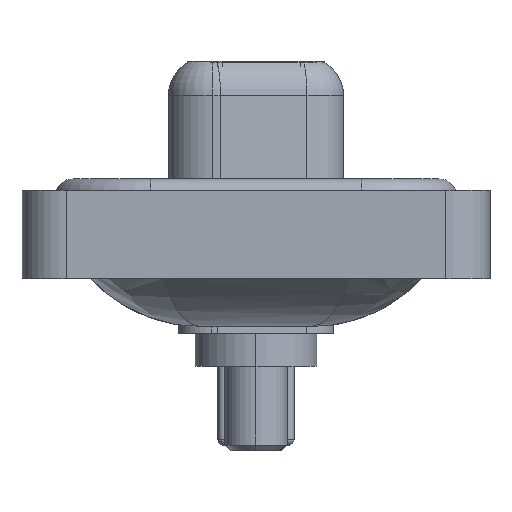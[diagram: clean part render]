
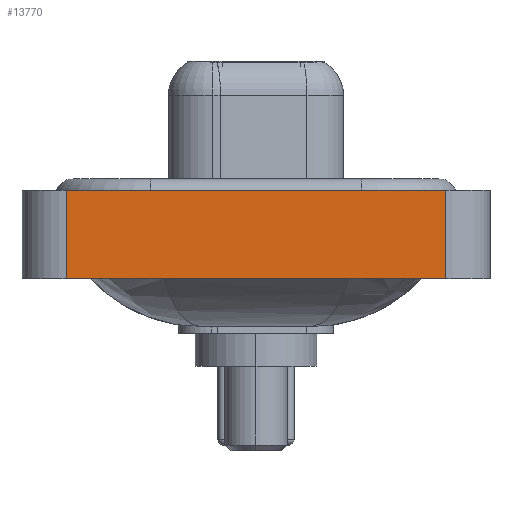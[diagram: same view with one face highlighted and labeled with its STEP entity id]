
A CAD part, left-side view. The second image highlights one B-rep face of the part: STEP entity #13770.
In plain terms, the highlighted planar face has unit normal (-1, 0, 0).
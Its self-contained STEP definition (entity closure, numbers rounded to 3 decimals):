
#622 = EDGE_CURVE ( 'NONE', #10113, #8779, #14927, .T. ) ;
#1394 = DIRECTION ( 'NONE',  ( 0., -1., 0. ) ) ;
#2522 = DIRECTION ( 'NONE',  ( -1., 0., 0. ) ) ;
#2656 = CARTESIAN_POINT ( 'NONE',  ( -7.35, -8.55, -3.6 ) ) ;
#2836 = DIRECTION ( 'NONE',  ( 0., -1., 0. ) ) ;
#3426 = VECTOR ( 'NONE', #14738, 1000. ) ;
#4171 = CARTESIAN_POINT ( 'NONE',  ( -7.35, 8.55, -3.6 ) ) ;
#4518 = ORIENTED_EDGE ( 'NONE', *, *, #9987, .F. ) ;
#4625 = CARTESIAN_POINT ( 'NONE',  ( -7.35, -8.55, -3.6 ) ) ;
#4740 = VECTOR ( 'NONE', #2836, 1000. ) ;
#5645 = PLANE ( 'NONE',  #9687 ) ;
#6592 = ORIENTED_EDGE ( 'NONE', *, *, #15192, .T. ) ;
#7659 = CARTESIAN_POINT ( 'NONE',  ( -7.35, -8.55, 0.4 ) ) ;
#7701 = ORIENTED_EDGE ( 'NONE', *, *, #15944, .F. ) ;
#7903 = CARTESIAN_POINT ( 'NONE',  ( -7.35, 8.55, 0.4 ) ) ;
#8779 = VERTEX_POINT ( 'NONE', #11919 ) ;
#8783 = VECTOR ( 'NONE', #1394, 1000. ) ;
#8885 = DIRECTION ( 'NONE',  ( 0., 0., 1. ) ) ;
#9007 = VERTEX_POINT ( 'NONE', #4171 ) ;
#9687 = AXIS2_PLACEMENT_3D ( 'NONE', #16875, #2522, #8885 ) ;
#9906 = LINE ( 'NONE', #16318, #3426 ) ;
#9987 = EDGE_CURVE ( 'NONE', #17891, #8779, #17233, .T. ) ;
#10113 = VERTEX_POINT ( 'NONE', #4625 ) ;
#10710 = VECTOR ( 'NONE', #14064, 1000. ) ;
#11919 = CARTESIAN_POINT ( 'NONE',  ( -7.35, -8.55, 0.4 ) ) ;
#12295 = EDGE_LOOP ( 'NONE', ( #16329, #4518, #7701, #6592 ) ) ;
#12345 = CARTESIAN_POINT ( 'NONE',  ( -7.35, -8.55, -3.6 ) ) ;
#13770 = ADVANCED_FACE ( 'NONE', ( #20008 ), #5645, .T. ) ;
#14064 = DIRECTION ( 'NONE',  ( 0., 0., 1. ) ) ;
#14738 = DIRECTION ( 'NONE',  ( 0., 0., 1. ) ) ;
#14927 = LINE ( 'NONE', #2656, #10710 ) ;
#15192 = EDGE_CURVE ( 'NONE', #9007, #10113, #17197, .T. ) ;
#15944 = EDGE_CURVE ( 'NONE', #9007, #17891, #9906, .T. ) ;
#16318 = CARTESIAN_POINT ( 'NONE',  ( -7.35, 8.55, -3.6 ) ) ;
#16329 = ORIENTED_EDGE ( 'NONE', *, *, #622, .T. ) ;
#16875 = CARTESIAN_POINT ( 'NONE',  ( -7.35, -8.55, -3.6 ) ) ;
#17197 = LINE ( 'NONE', #12345, #4740 ) ;
#17233 = LINE ( 'NONE', #7659, #8783 ) ;
#17891 = VERTEX_POINT ( 'NONE', #7903 ) ;
#20008 = FACE_OUTER_BOUND ( 'NONE', #12295, .T. ) ;
